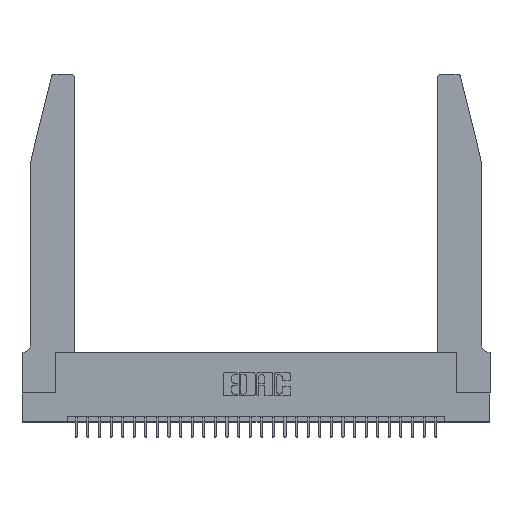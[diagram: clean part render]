
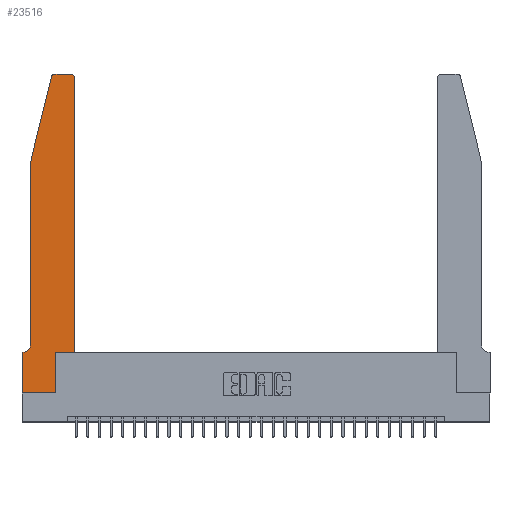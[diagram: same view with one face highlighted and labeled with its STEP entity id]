
A CAD part, top view. The second image highlights one B-rep face of the part: STEP entity #23516.
In plain terms, the highlighted planar face has unit normal (0, 0, 1).
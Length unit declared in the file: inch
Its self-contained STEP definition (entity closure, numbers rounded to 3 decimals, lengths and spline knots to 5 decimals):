
#233 = EDGE_CURVE ( 'NONE', #22089, #13972, #20918, .T. ) ;
#602 = PLANE ( 'NONE',  #15306 ) ;
#879 = CARTESIAN_POINT ( 'NONE',  ( 0.4205, 2.72, 0.37 ) ) ;
#929 = EDGE_CURVE ( 'NONE', #18222, #25575, #21808, .T. ) ;
#1239 = ORIENTED_EDGE ( 'NONE', *, *, #24925, .T. ) ;
#1338 = CARTESIAN_POINT ( 'NONE',  ( 0.0055, 0.35, 0.37 ) ) ;
#1353 = DIRECTION ( 'NONE',  ( 0., 0., 1. ) ) ;
#2323 = CARTESIAN_POINT ( 'NONE',  ( 0.0755, 2., 0.37 ) ) ;
#3287 = CARTESIAN_POINT ( 'NONE',  ( 0.0755, 2., 0.37 ) ) ;
#3767 = DIRECTION ( 'NONE',  ( 0., 0., 1. ) ) ;
#4213 = ORIENTED_EDGE ( 'NONE', *, *, #233, .T. ) ;
#4240 = CARTESIAN_POINT ( 'NONE',  ( 0.2865, 0.35, 0.37 ) ) ;
#4532 = VECTOR ( 'NONE', #24652, 39.37008 ) ;
#4698 = ORIENTED_EDGE ( 'NONE', *, *, #26990, .T. ) ;
#4824 = ORIENTED_EDGE ( 'NONE', *, *, #24075, .T. ) ;
#4850 = DIRECTION ( 'NONE',  ( 0., -1., 0. ) ) ;
#4882 = DIRECTION ( 'NONE',  ( 1., 0., 0. ) ) ;
#5327 = VERTEX_POINT ( 'NONE', #13806 ) ;
#5400 = VECTOR ( 'NONE', #14252, 39.37008 ) ;
#5640 = EDGE_CURVE ( 'NONE', #25575, #16014, #29770, .T. ) ;
#6144 = CARTESIAN_POINT ( 'NONE',  ( 0.25487, 2.72718, 0.37 ) ) ;
#6305 = LINE ( 'NONE', #30553, #5400 ) ;
#6432 = VERTEX_POINT ( 'NONE', #23354 ) ;
#6524 = LINE ( 'NONE', #30137, #16273 ) ;
#6946 = VERTEX_POINT ( 'NONE', #6144 ) ;
#7270 = DIRECTION ( 'NONE',  ( 0., 0., 1. ) ) ;
#7411 = VERTEX_POINT ( 'NONE', #18174 ) ;
#7651 = AXIS2_PLACEMENT_3D ( 'NONE', #8738, #28539, #25981 ) ;
#7887 = LINE ( 'NONE', #3287, #17522 ) ;
#8527 = DIRECTION ( 'NONE',  ( 1., 0., 0. ) ) ;
#8738 = CARTESIAN_POINT ( 'NONE',  ( 0.0055, 0.42, 0.37 ) ) ;
#10217 = ORIENTED_EDGE ( 'NONE', *, *, #15976, .T. ) ;
#10935 = CARTESIAN_POINT ( 'NONE',  ( 0.2605, 2.75, 0.37 ) ) ;
#13232 = CIRCLE ( 'NONE', #17266, 0.03 ) ;
#13476 = CARTESIAN_POINT ( 'NONE',  ( 0., 0., 0.37 ) ) ;
#13806 = CARTESIAN_POINT ( 'NONE',  ( 0., 0.35, 0.37 ) ) ;
#13972 = VERTEX_POINT ( 'NONE', #30927 ) ;
#14184 = EDGE_LOOP ( 'NONE', ( #23932, #1239, #28657, #10217, #28142, #4824, #30551, #15591, #20966, #4698, #4213, #21270 ) ) ;
#14252 = DIRECTION ( 'NONE',  ( 0., -1., 0. ) ) ;
#14467 = EDGE_CURVE ( 'NONE', #6946, #7411, #7887, .T. ) ;
#15306 = AXIS2_PLACEMENT_3D ( 'NONE', #28994, #7270, #4882 ) ;
#15375 = CARTESIAN_POINT ( 'NONE',  ( 0.2865, 0.35, 0.37 ) ) ;
#15535 = DIRECTION ( 'NONE',  ( -1., 0., 0. ) ) ;
#15591 = ORIENTED_EDGE ( 'NONE', *, *, #929, .T. ) ;
#15796 = EDGE_CURVE ( 'NONE', #16343, #6432, #20879, .T. ) ;
#15867 = EDGE_CURVE ( 'NONE', #5327, #18222, #6305, .T. ) ;
#15976 = EDGE_CURVE ( 'NONE', #7411, #29893, #26254, .T. ) ;
#16014 = VERTEX_POINT ( 'NONE', #4240 ) ;
#16067 = DIRECTION ( 'NONE',  ( -1., 0., 0. ) ) ;
#16273 = VECTOR ( 'NONE', #16067, 39.37008 ) ;
#16343 = VERTEX_POINT ( 'NONE', #24120 ) ;
#16577 = CARTESIAN_POINT ( 'NONE',  ( 0.2865, 0., 0.37 ) ) ;
#17266 = AXIS2_PLACEMENT_3D ( 'NONE', #25620, #3767, #8527 ) ;
#17343 = DIRECTION ( 'NONE',  ( 1., 0., 0. ) ) ;
#17494 = LINE ( 'NONE', #29392, #19386 ) ;
#17522 = VECTOR ( 'NONE', #17559, 39.37008 ) ;
#17559 = DIRECTION ( 'NONE',  ( -0.239, -0.971, 0. ) ) ;
#18174 = CARTESIAN_POINT ( 'NONE',  ( 0.0755, 2., 0.37 ) ) ;
#18222 = VERTEX_POINT ( 'NONE', #13476 ) ;
#18229 = DIRECTION ( 'NONE',  ( 0., 1., 0. ) ) ;
#18926 = VECTOR ( 'NONE', #26908, 39.37008 ) ;
#19080 = VECTOR ( 'NONE', #15535, 39.37008 ) ;
#19386 = VECTOR ( 'NONE', #17343, 39.37008 ) ;
#19899 = CARTESIAN_POINT ( 'NONE',  ( 0., 0., 0.37 ) ) ;
#20879 = LINE ( 'NONE', #10935, #19080 ) ;
#20918 = LINE ( 'NONE', #23128, #27286 ) ;
#20966 = ORIENTED_EDGE ( 'NONE', *, *, #5640, .T. ) ;
#21270 = ORIENTED_EDGE ( 'NONE', *, *, #26623, .T. ) ;
#21310 = CIRCLE ( 'NONE', #7651, 0.07 ) ;
#21808 = LINE ( 'NONE', #19899, #4532 ) ;
#21923 = CARTESIAN_POINT ( 'NONE',  ( 0.0755, 0.42, 0.37 ) ) ;
#22089 = VERTEX_POINT ( 'NONE', #28101 ) ;
#22305 = FACE_OUTER_BOUND ( 'NONE', #14184, .T. ) ;
#22396 = EDGE_CURVE ( 'NONE', #29893, #28486, #21310, .T. ) ;
#23128 = CARTESIAN_POINT ( 'NONE',  ( 0.4505, 0.35, 0.37 ) ) ;
#23354 = CARTESIAN_POINT ( 'NONE',  ( 0.284, 2.75, 0.37 ) ) ;
#23423 = CIRCLE ( 'NONE', #30017, 0.03 ) ;
#23516 = ADVANCED_FACE ( 'NONE', ( #22305 ), #602, .T. ) ;
#23932 = ORIENTED_EDGE ( 'NONE', *, *, #15796, .T. ) ;
#24075 = EDGE_CURVE ( 'NONE', #28486, #5327, #6524, .T. ) ;
#24120 = CARTESIAN_POINT ( 'NONE',  ( 0.4205, 2.75, 0.37 ) ) ;
#24652 = DIRECTION ( 'NONE',  ( 1., 0., 0. ) ) ;
#24925 = EDGE_CURVE ( 'NONE', #6432, #6946, #13232, .T. ) ;
#25575 = VERTEX_POINT ( 'NONE', #16577 ) ;
#25620 = CARTESIAN_POINT ( 'NONE',  ( 0.284, 2.72, 0.37 ) ) ;
#25981 = DIRECTION ( 'NONE',  ( -1., 0., 0. ) ) ;
#26254 = LINE ( 'NONE', #2323, #28196 ) ;
#26623 = EDGE_CURVE ( 'NONE', #13972, #16343, #23423, .T. ) ;
#26908 = DIRECTION ( 'NONE',  ( 0., 1., 0. ) ) ;
#26990 = EDGE_CURVE ( 'NONE', #16014, #22089, #17494, .T. ) ;
#27286 = VECTOR ( 'NONE', #18229, 39.37008 ) ;
#27349 = DIRECTION ( 'NONE',  ( 1., 0., 0. ) ) ;
#28101 = CARTESIAN_POINT ( 'NONE',  ( 0.4505, 0.35, 0.37 ) ) ;
#28142 = ORIENTED_EDGE ( 'NONE', *, *, #22396, .T. ) ;
#28196 = VECTOR ( 'NONE', #4850, 39.37008 ) ;
#28486 = VERTEX_POINT ( 'NONE', #1338 ) ;
#28539 = DIRECTION ( 'NONE',  ( 0., 0., -1. ) ) ;
#28657 = ORIENTED_EDGE ( 'NONE', *, *, #14467, .T. ) ;
#28994 = CARTESIAN_POINT ( 'NONE',  ( 0., 0.35, 0.37 ) ) ;
#29392 = CARTESIAN_POINT ( 'NONE',  ( 0.4505, 0.35, 0.37 ) ) ;
#29770 = LINE ( 'NONE', #15375, #18926 ) ;
#29893 = VERTEX_POINT ( 'NONE', #21923 ) ;
#30017 = AXIS2_PLACEMENT_3D ( 'NONE', #879, #1353, #27349 ) ;
#30137 = CARTESIAN_POINT ( 'NONE',  ( 0.0755, 0.35, 0.37 ) ) ;
#30551 = ORIENTED_EDGE ( 'NONE', *, *, #15867, .T. ) ;
#30553 = CARTESIAN_POINT ( 'NONE',  ( 0., 0., 0.37 ) ) ;
#30927 = CARTESIAN_POINT ( 'NONE',  ( 0.4505, 2.72, 0.37 ) ) ;
